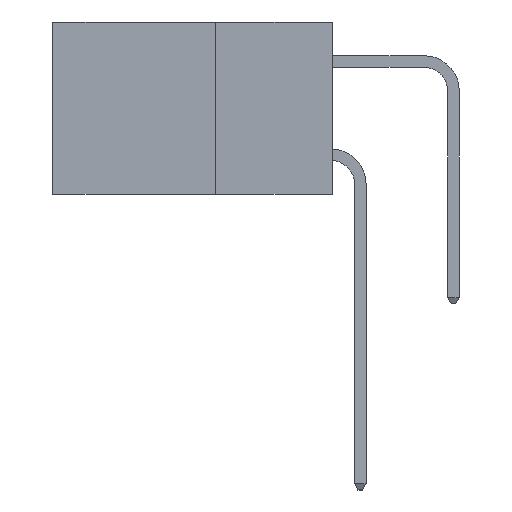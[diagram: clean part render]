
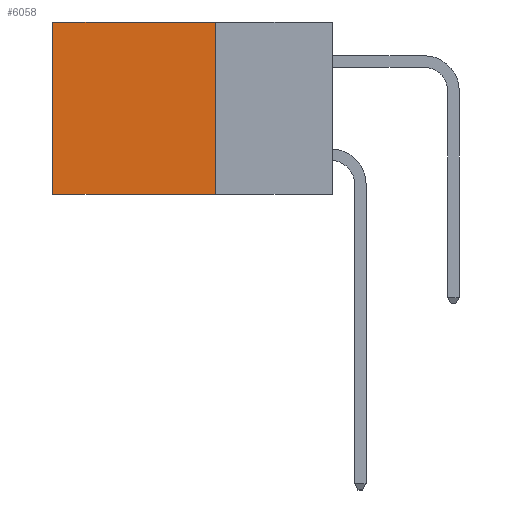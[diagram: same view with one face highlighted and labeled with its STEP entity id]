
A CAD part, left-side view. The second image highlights one B-rep face of the part: STEP entity #6058.
In plain terms, the highlighted planar face has unit normal (-1, 0, 0).
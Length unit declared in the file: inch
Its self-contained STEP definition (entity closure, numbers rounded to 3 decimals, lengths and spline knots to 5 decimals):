
#845 = LINE ( 'NONE', #9968, #6139 ) ;
#1344 = VERTEX_POINT ( 'NONE', #2380 ) ;
#1362 = CARTESIAN_POINT ( 'NONE',  ( 0.2615, 0.6, 0. ) ) ;
#1464 = CARTESIAN_POINT ( 'NONE',  ( 0.2615, 0.25, -0.37 ) ) ;
#1611 = EDGE_CURVE ( 'NONE', #5915, #1344, #12230, .T. ) ;
#2124 = VECTOR ( 'NONE', #9568, 39.37008 ) ;
#2167 = ORIENTED_EDGE ( 'NONE', *, *, #6001, .F. ) ;
#2288 = EDGE_CURVE ( 'NONE', #4009, #8427, #10266, .T. ) ;
#2380 = CARTESIAN_POINT ( 'NONE',  ( 0.2615, 0.25, -0.37 ) ) ;
#2426 = DIRECTION ( 'NONE',  ( 0., 0., -1. ) ) ;
#2981 = CARTESIAN_POINT ( 'NONE',  ( 0.2615, 0.25, 0. ) ) ;
#3326 = CARTESIAN_POINT ( 'NONE',  ( 0.2615, 0.25, 0. ) ) ;
#3408 = DIRECTION ( 'NONE',  ( 0., 1., 0. ) ) ;
#3413 = CARTESIAN_POINT ( 'NONE',  ( 0.2615, 0.25, -0.37 ) ) ;
#3478 = ORIENTED_EDGE ( 'NONE', *, *, #1611, .F. ) ;
#3486 = DIRECTION ( 'NONE',  ( 0., 0., -1. ) ) ;
#4009 = VERTEX_POINT ( 'NONE', #1362 ) ;
#4410 = PLANE ( 'NONE',  #8383 ) ;
#4419 = LINE ( 'NONE', #2981, #2124 ) ;
#4599 = ORIENTED_EDGE ( 'NONE', *, *, #2288, .T. ) ;
#4999 = EDGE_LOOP ( 'NONE', ( #4599, #2167, #3478, #10074 ) ) ;
#5297 = VECTOR ( 'NONE', #11993, 39.37008 ) ;
#5507 = FACE_OUTER_BOUND ( 'NONE', #4999, .T. ) ;
#5915 = VERTEX_POINT ( 'NONE', #3326 ) ;
#6001 = EDGE_CURVE ( 'NONE', #1344, #8427, #845, .T. ) ;
#6058 = ADVANCED_FACE ( 'NONE', ( #5507 ), #4410, .F. ) ;
#6139 = VECTOR ( 'NONE', #3408, 39.37008 ) ;
#8383 = AXIS2_PLACEMENT_3D ( 'NONE', #1464, #9157, #3486 ) ;
#8427 = VERTEX_POINT ( 'NONE', #9548 ) ;
#9157 = DIRECTION ( 'NONE',  ( 1., 0., 0. ) ) ;
#9548 = CARTESIAN_POINT ( 'NONE',  ( 0.2615, 0.6, -0.37 ) ) ;
#9568 = DIRECTION ( 'NONE',  ( 0., 1., 0. ) ) ;
#9861 = VECTOR ( 'NONE', #2426, 39.37008 ) ;
#9968 = CARTESIAN_POINT ( 'NONE',  ( 0.2615, 0.25, -0.37 ) ) ;
#10074 = ORIENTED_EDGE ( 'NONE', *, *, #10585, .T. ) ;
#10266 = LINE ( 'NONE', #12007, #5297 ) ;
#10585 = EDGE_CURVE ( 'NONE', #5915, #4009, #4419, .T. ) ;
#11993 = DIRECTION ( 'NONE',  ( 0., 0., -1. ) ) ;
#12007 = CARTESIAN_POINT ( 'NONE',  ( 0.2615, 0.6, -0.37 ) ) ;
#12230 = LINE ( 'NONE', #3413, #9861 ) ;
